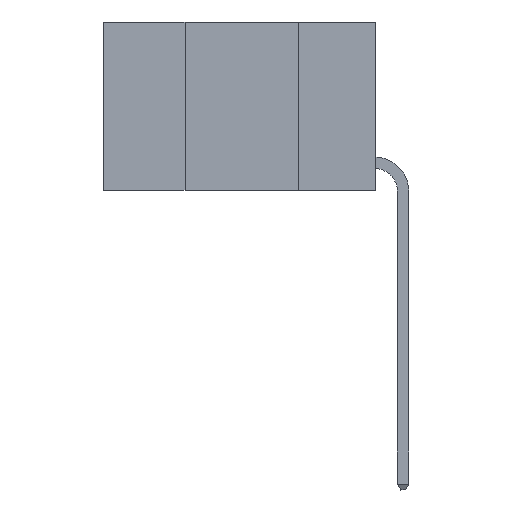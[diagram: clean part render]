
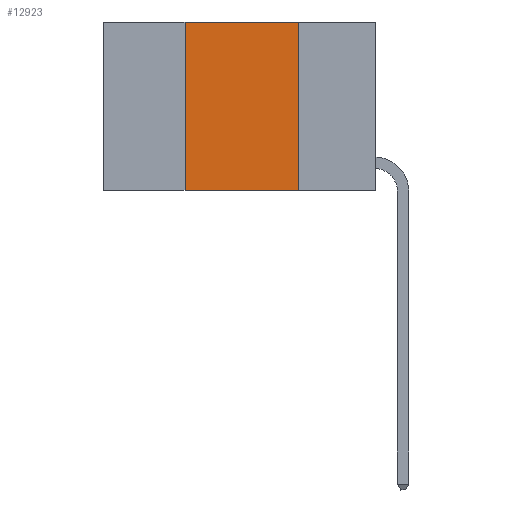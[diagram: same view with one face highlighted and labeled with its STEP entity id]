
A CAD part, left-side view. The second image highlights one B-rep face of the part: STEP entity #12923.
In plain terms, the highlighted planar face has unit normal (-1, 0, 0).
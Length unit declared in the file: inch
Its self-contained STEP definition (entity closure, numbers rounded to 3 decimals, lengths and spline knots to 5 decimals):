
#48 = DIRECTION ( 'NONE',  ( 0., -1., 0. ) ) ;
#451 = EDGE_CURVE ( 'NONE', #16780, #15847, #10102, .T. ) ;
#525 = ORIENTED_EDGE ( 'NONE', *, *, #14479, .T. ) ;
#750 = AXIS2_PLACEMENT_3D ( 'NONE', #11192, #16775, #3978 ) ;
#1082 = ORIENTED_EDGE ( 'NONE', *, *, #17805, .F. ) ;
#1657 = CARTESIAN_POINT ( 'NONE',  ( 0., 0.42, 0. ) ) ;
#2026 = EDGE_LOOP ( 'NONE', ( #14915, #3148, #1082, #525 ) ) ;
#2835 = VECTOR ( 'NONE', #18397, 39.37008 ) ;
#3148 = ORIENTED_EDGE ( 'NONE', *, *, #451, .F. ) ;
#3508 = CARTESIAN_POINT ( 'NONE',  ( 0., 0.17, 0. ) ) ;
#3978 = DIRECTION ( 'NONE',  ( 0., 0., -1. ) ) ;
#4513 = LINE ( 'NONE', #1657, #6604 ) ;
#4544 = CARTESIAN_POINT ( 'NONE',  ( 0., 0.17, -0.37 ) ) ;
#5167 = VERTEX_POINT ( 'NONE', #4544 ) ;
#5785 = VERTEX_POINT ( 'NONE', #7141 ) ;
#5986 = EDGE_CURVE ( 'NONE', #15847, #5167, #9413, .T. ) ;
#6167 = DIRECTION ( 'NONE',  ( 0., -1., 0. ) ) ;
#6604 = VECTOR ( 'NONE', #10301, 39.37008 ) ;
#6659 = CARTESIAN_POINT ( 'NONE',  ( 0., 0.17, 0. ) ) ;
#7141 = CARTESIAN_POINT ( 'NONE',  ( 0., 0.42, -0.37 ) ) ;
#9413 = LINE ( 'NONE', #6659, #2835 ) ;
#9497 = PLANE ( 'NONE',  #750 ) ;
#10102 = LINE ( 'NONE', #15857, #13438 ) ;
#10301 = DIRECTION ( 'NONE',  ( 0., 0., 1. ) ) ;
#10532 = LINE ( 'NONE', #12046, #12597 ) ;
#11192 = CARTESIAN_POINT ( 'NONE',  ( 0., 0.6, 0. ) ) ;
#12046 = CARTESIAN_POINT ( 'NONE',  ( 0., 0.6, -0.37 ) ) ;
#12597 = VECTOR ( 'NONE', #6167, 39.37008 ) ;
#12605 = FACE_OUTER_BOUND ( 'NONE', #2026, .T. ) ;
#12923 = ADVANCED_FACE ( 'NONE', ( #12605 ), #9497, .F. ) ;
#13438 = VECTOR ( 'NONE', #48, 39.37008 ) ;
#14479 = EDGE_CURVE ( 'NONE', #5785, #5167, #10532, .T. ) ;
#14915 = ORIENTED_EDGE ( 'NONE', *, *, #5986, .F. ) ;
#15847 = VERTEX_POINT ( 'NONE', #3508 ) ;
#15857 = CARTESIAN_POINT ( 'NONE',  ( 0., 0.6, 0. ) ) ;
#16775 = DIRECTION ( 'NONE',  ( 1., 0., 0. ) ) ;
#16780 = VERTEX_POINT ( 'NONE', #18033 ) ;
#17805 = EDGE_CURVE ( 'NONE', #5785, #16780, #4513, .T. ) ;
#18033 = CARTESIAN_POINT ( 'NONE',  ( 0., 0.42, 0. ) ) ;
#18397 = DIRECTION ( 'NONE',  ( 0., 0., -1. ) ) ;
